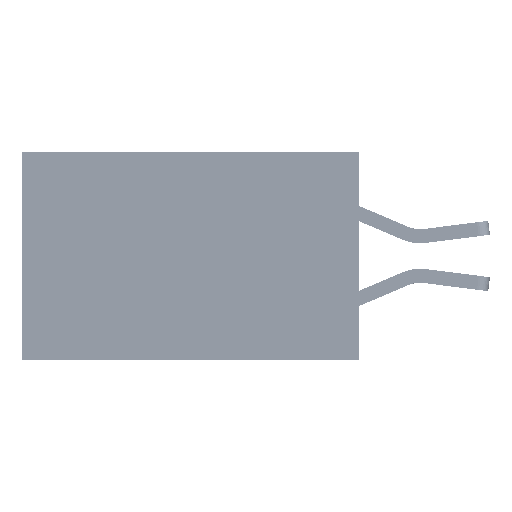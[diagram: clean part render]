
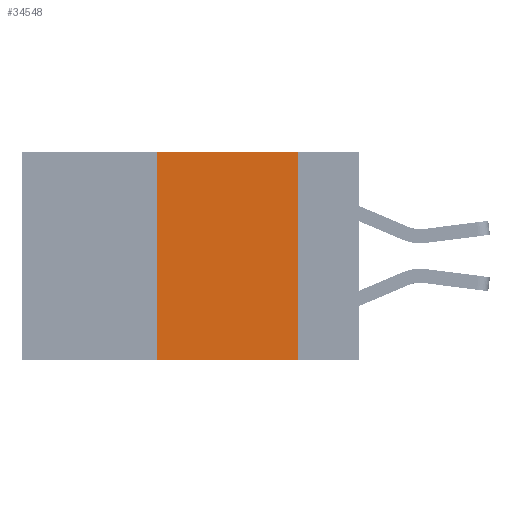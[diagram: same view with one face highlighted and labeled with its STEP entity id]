
A CAD part, left-side view. The second image highlights one B-rep face of the part: STEP entity #34548.
In plain terms, the highlighted planar face has unit normal (-1, 0, 0).
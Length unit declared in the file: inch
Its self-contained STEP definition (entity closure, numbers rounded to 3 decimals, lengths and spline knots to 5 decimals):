
#2830 = VERTEX_POINT ( 'NONE', #8578 ) ;
#3394 = LINE ( 'NONE', #18705, #45714 ) ;
#4584 = DIRECTION ( 'NONE',  ( 1., 0., 0. ) ) ;
#4829 = CARTESIAN_POINT ( 'NONE',  ( 0., 0.6, 0. ) ) ;
#5194 = VERTEX_POINT ( 'NONE', #14133 ) ;
#6122 = CARTESIAN_POINT ( 'NONE',  ( 0., 0.11, 0. ) ) ;
#8578 = CARTESIAN_POINT ( 'NONE',  ( 0., 0.11, -0.37 ) ) ;
#10517 = VECTOR ( 'NONE', #28964, 39.37008 ) ;
#14133 = CARTESIAN_POINT ( 'NONE',  ( 0., 0.36, 0. ) ) ;
#16557 = EDGE_CURVE ( 'NONE', #5194, #20324, #32190, .T. ) ;
#17744 = LINE ( 'NONE', #32357, #27341 ) ;
#18705 = CARTESIAN_POINT ( 'NONE',  ( 0., 0.36, 0. ) ) ;
#20324 = VERTEX_POINT ( 'NONE', #6122 ) ;
#20359 = EDGE_CURVE ( 'NONE', #20324, #2830, #17744, .T. ) ;
#20527 = EDGE_LOOP ( 'NONE', ( #28278, #48586, #30719, #23366 ) ) ;
#21532 = CARTESIAN_POINT ( 'NONE',  ( 0., 0.6, 0. ) ) ;
#22636 = FACE_OUTER_BOUND ( 'NONE', #20527, .T. ) ;
#23366 = ORIENTED_EDGE ( 'NONE', *, *, #32444, .T. ) ;
#24523 = AXIS2_PLACEMENT_3D ( 'NONE', #4829, #4584, #41452 ) ;
#27341 = VECTOR ( 'NONE', #40267, 39.37008 ) ;
#27780 = CARTESIAN_POINT ( 'NONE',  ( 0., 0.6, -0.37 ) ) ;
#28278 = ORIENTED_EDGE ( 'NONE', *, *, #20359, .F. ) ;
#28964 = DIRECTION ( 'NONE',  ( 0., -1., 0. ) ) ;
#30194 = EDGE_CURVE ( 'NONE', #35244, #5194, #3394, .T. ) ;
#30719 = ORIENTED_EDGE ( 'NONE', *, *, #30194, .F. ) ;
#32190 = LINE ( 'NONE', #21532, #10517 ) ;
#32357 = CARTESIAN_POINT ( 'NONE',  ( 0., 0.11, 0. ) ) ;
#32444 = EDGE_CURVE ( 'NONE', #35244, #2830, #47056, .T. ) ;
#34548 = ADVANCED_FACE ( 'NONE', ( #22636 ), #38228, .F. ) ;
#35244 = VERTEX_POINT ( 'NONE', #47535 ) ;
#37026 = DIRECTION ( 'NONE',  ( 0., 0., 1. ) ) ;
#38228 = PLANE ( 'NONE',  #24523 ) ;
#39155 = DIRECTION ( 'NONE',  ( 0., -1., 0. ) ) ;
#40267 = DIRECTION ( 'NONE',  ( 0., 0., -1. ) ) ;
#41452 = DIRECTION ( 'NONE',  ( 0., 0., -1. ) ) ;
#44155 = VECTOR ( 'NONE', #39155, 39.37008 ) ;
#45714 = VECTOR ( 'NONE', #37026, 39.37008 ) ;
#47056 = LINE ( 'NONE', #27780, #44155 ) ;
#47535 = CARTESIAN_POINT ( 'NONE',  ( 0., 0.36, -0.37 ) ) ;
#48586 = ORIENTED_EDGE ( 'NONE', *, *, #16557, .F. ) ;
